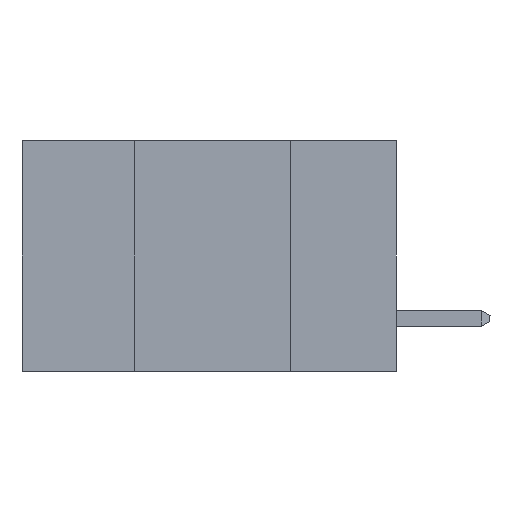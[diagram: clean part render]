
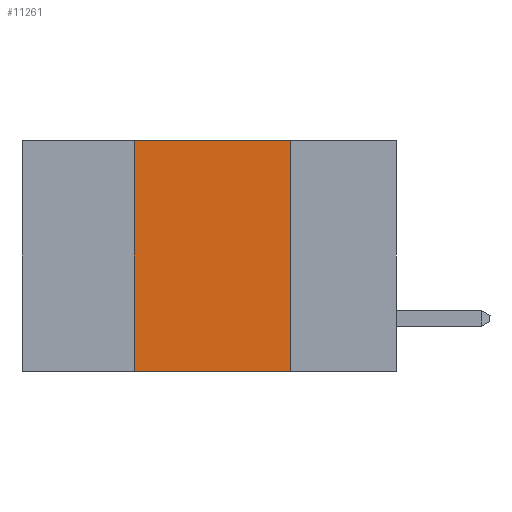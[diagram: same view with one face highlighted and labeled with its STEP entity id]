
A CAD part, left-side view. The second image highlights one B-rep face of the part: STEP entity #11261.
In plain terms, the highlighted planar face has unit normal (-1, 0, 0).
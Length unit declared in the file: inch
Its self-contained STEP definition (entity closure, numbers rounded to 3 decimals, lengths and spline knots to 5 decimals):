
#255 = VECTOR ( 'NONE', #14826, 39.37008 ) ;
#730 = CARTESIAN_POINT ( 'NONE',  ( 0., 0.42, 0. ) ) ;
#1693 = VECTOR ( 'NONE', #9982, 39.37008 ) ;
#1847 = DIRECTION ( 'NONE',  ( 1., 0., 0. ) ) ;
#2443 = AXIS2_PLACEMENT_3D ( 'NONE', #12581, #1847, #5819 ) ;
#2455 = VERTEX_POINT ( 'NONE', #11209 ) ;
#3016 = FACE_OUTER_BOUND ( 'NONE', #11300, .T. ) ;
#3056 = CARTESIAN_POINT ( 'NONE',  ( 0., 0.17, -0.37 ) ) ;
#3267 = EDGE_CURVE ( 'NONE', #15464, #4787, #13187, .T. ) ;
#4003 = LINE ( 'NONE', #3056, #1693 ) ;
#4434 = CARTESIAN_POINT ( 'NONE',  ( 0., 0.6, 0. ) ) ;
#4787 = VERTEX_POINT ( 'NONE', #730 ) ;
#4805 = VECTOR ( 'NONE', #6053, 39.37008 ) ;
#5025 = CARTESIAN_POINT ( 'NONE',  ( 0., 0.42, -0.37 ) ) ;
#5819 = DIRECTION ( 'NONE',  ( 0., 0., -1. ) ) ;
#6053 = DIRECTION ( 'NONE',  ( 0., 0., 1. ) ) ;
#7803 = PLANE ( 'NONE',  #2443 ) ;
#8091 = ORIENTED_EDGE ( 'NONE', *, *, #12624, .T. ) ;
#8990 = EDGE_CURVE ( 'NONE', #4787, #2455, #10134, .T. ) ;
#9982 = DIRECTION ( 'NONE',  ( 0., 0., -1. ) ) ;
#9998 = LINE ( 'NONE', #11158, #255 ) ;
#10134 = LINE ( 'NONE', #4434, #13172 ) ;
#10165 = EDGE_CURVE ( 'NONE', #2455, #14734, #4003, .T. ) ;
#11158 = CARTESIAN_POINT ( 'NONE',  ( 0., 0.6, -0.37 ) ) ;
#11209 = CARTESIAN_POINT ( 'NONE',  ( 0., 0.17, 0. ) ) ;
#11261 = ADVANCED_FACE ( 'NONE', ( #3016 ), #7803, .F. ) ;
#11300 = EDGE_LOOP ( 'NONE', ( #14247, #13154, #12918, #8091 ) ) ;
#12581 = CARTESIAN_POINT ( 'NONE',  ( 0., 0.6, 0. ) ) ;
#12624 = EDGE_CURVE ( 'NONE', #15464, #14734, #9998, .T. ) ;
#12918 = ORIENTED_EDGE ( 'NONE', *, *, #3267, .F. ) ;
#13154 = ORIENTED_EDGE ( 'NONE', *, *, #8990, .F. ) ;
#13172 = VECTOR ( 'NONE', #14889, 39.37008 ) ;
#13187 = LINE ( 'NONE', #5025, #4805 ) ;
#13551 = CARTESIAN_POINT ( 'NONE',  ( 0., 0.17, -0.37 ) ) ;
#14247 = ORIENTED_EDGE ( 'NONE', *, *, #10165, .F. ) ;
#14717 = CARTESIAN_POINT ( 'NONE',  ( 0., 0.42, -0.37 ) ) ;
#14734 = VERTEX_POINT ( 'NONE', #13551 ) ;
#14826 = DIRECTION ( 'NONE',  ( 0., -1., 0. ) ) ;
#14889 = DIRECTION ( 'NONE',  ( 0., -1., 0. ) ) ;
#15464 = VERTEX_POINT ( 'NONE', #14717 ) ;
